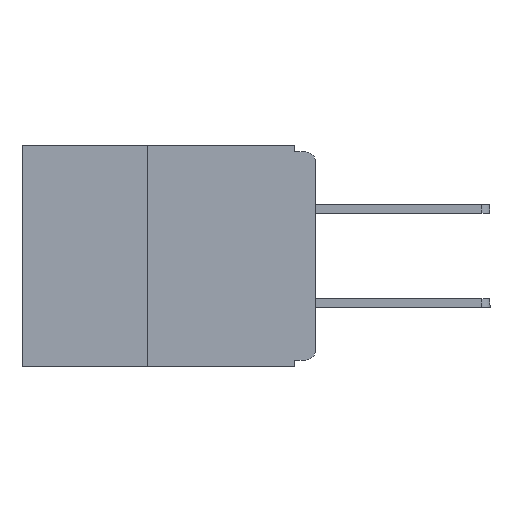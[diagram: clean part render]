
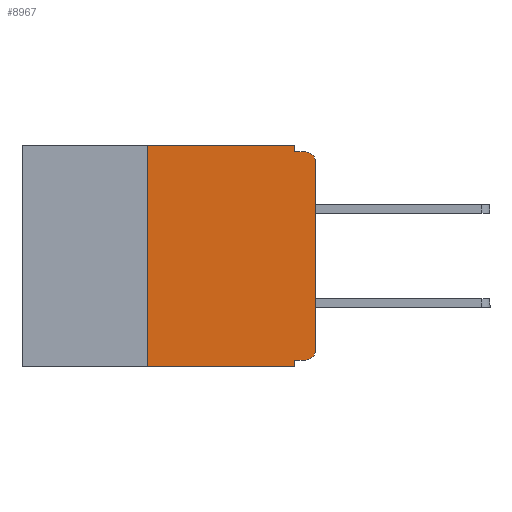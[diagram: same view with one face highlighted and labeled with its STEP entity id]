
A CAD part, left-side view. The second image highlights one B-rep face of the part: STEP entity #8967.
In plain terms, the highlighted planar face has unit normal (-1, 0, 0).
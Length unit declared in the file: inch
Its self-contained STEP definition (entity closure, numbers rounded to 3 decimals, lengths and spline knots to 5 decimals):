
#3 = VERTEX_POINT ( 'NONE', #2808 ) ;
#94 = DIRECTION ( 'NONE',  ( 0., -1., 0. ) ) ;
#122 = CARTESIAN_POINT ( 'NONE',  ( 0., 0.015, -0.01 ) ) ;
#172 = ORIENTED_EDGE ( 'NONE', *, *, #10908, .F. ) ;
#770 = EDGE_CURVE ( 'NONE', #8113, #10541, #4836, .T. ) ;
#774 = EDGE_CURVE ( 'NONE', #13539, #8169, #15194, .T. ) ;
#824 = CIRCLE ( 'NONE', #11983, 0.015 ) ;
#1179 = VECTOR ( 'NONE', #11630, 39.37008 ) ;
#1197 = EDGE_CURVE ( 'NONE', #11318, #4646, #5446, .T. ) ;
#1811 = VECTOR ( 'NONE', #4163, 39.37008 ) ;
#1827 = CARTESIAN_POINT ( 'NONE',  ( 0., 0.015, -0.32 ) ) ;
#2055 = EDGE_LOOP ( 'NONE', ( #10317, #3755, #13589, #3401, #172, #10776, #5014, #6079, #3906, #14213 ) ) ;
#2727 = CARTESIAN_POINT ( 'NONE',  ( 0., 0.015, -0.305 ) ) ;
#2808 = CARTESIAN_POINT ( 'NONE',  ( 0., 0.031, 0. ) ) ;
#3328 = CARTESIAN_POINT ( 'NONE',  ( 0., 0.031, -0.32 ) ) ;
#3401 = ORIENTED_EDGE ( 'NONE', *, *, #4735, .F. ) ;
#3531 = CARTESIAN_POINT ( 'NONE',  ( 0., 0.25, -0.33 ) ) ;
#3652 = EDGE_CURVE ( 'NONE', #11318, #11875, #12510, .T. ) ;
#3719 = EDGE_CURVE ( 'NONE', #10541, #15832, #824, .T. ) ;
#3755 = ORIENTED_EDGE ( 'NONE', *, *, #3719, .T. ) ;
#3906 = ORIENTED_EDGE ( 'NONE', *, *, #774, .F. ) ;
#4073 = DIRECTION ( 'NONE',  ( 0., 0., -1. ) ) ;
#4163 = DIRECTION ( 'NONE',  ( 0., 0., 1. ) ) ;
#4646 = VERTEX_POINT ( 'NONE', #12710 ) ;
#4735 = EDGE_CURVE ( 'NONE', #3, #14463, #13981, .T. ) ;
#4836 = LINE ( 'NONE', #10159, #1179 ) ;
#5014 = ORIENTED_EDGE ( 'NONE', *, *, #3652, .T. ) ;
#5231 = LINE ( 'NONE', #16571, #11992 ) ;
#5446 = LINE ( 'NONE', #3531, #1811 ) ;
#5982 = EDGE_CURVE ( 'NONE', #8169, #11875, #5231, .T. ) ;
#6079 = ORIENTED_EDGE ( 'NONE', *, *, #5982, .F. ) ;
#6675 = DIRECTION ( 'NONE',  ( 0., 0., -1. ) ) ;
#7108 = CARTESIAN_POINT ( 'NONE',  ( 0., 0., -0.025 ) ) ;
#7160 = CARTESIAN_POINT ( 'NONE',  ( 0., 0.031, 0. ) ) ;
#7494 = CARTESIAN_POINT ( 'NONE',  ( 0., 0., -0.305 ) ) ;
#7818 = CARTESIAN_POINT ( 'NONE',  ( 0., 0.031, -0.01 ) ) ;
#8113 = VERTEX_POINT ( 'NONE', #7494 ) ;
#8169 = VERTEX_POINT ( 'NONE', #3328 ) ;
#8844 = VECTOR ( 'NONE', #9784, 39.37008 ) ;
#8901 = VECTOR ( 'NONE', #9251, 39.37008 ) ;
#8906 = LINE ( 'NONE', #16285, #15675 ) ;
#8967 = ADVANCED_FACE ( 'NONE', ( #17340 ), #14447, .F. ) ;
#9251 = DIRECTION ( 'NONE',  ( 0., -1., 0. ) ) ;
#9534 = CIRCLE ( 'NONE', #13207, 0.015 ) ;
#9784 = DIRECTION ( 'NONE',  ( 0., 1., 0. ) ) ;
#9944 = VECTOR ( 'NONE', #6675, 39.37008 ) ;
#10095 = DIRECTION ( 'NONE',  ( 0., -1., 0. ) ) ;
#10159 = CARTESIAN_POINT ( 'NONE',  ( 0., 0., 0. ) ) ;
#10317 = ORIENTED_EDGE ( 'NONE', *, *, #770, .T. ) ;
#10467 = AXIS2_PLACEMENT_3D ( 'NONE', #14852, #14054, #14014 ) ;
#10541 = VERTEX_POINT ( 'NONE', #7108 ) ;
#10776 = ORIENTED_EDGE ( 'NONE', *, *, #1197, .F. ) ;
#10908 = EDGE_CURVE ( 'NONE', #4646, #3, #8906, .T. ) ;
#11052 = CARTESIAN_POINT ( 'NONE',  ( 0., 0.015, -0.025 ) ) ;
#11318 = VERTEX_POINT ( 'NONE', #13174 ) ;
#11333 = VECTOR ( 'NONE', #10095, 39.37008 ) ;
#11450 = DIRECTION ( 'NONE',  ( -1., 0., 0. ) ) ;
#11522 = CARTESIAN_POINT ( 'NONE',  ( 0., 0.031, -0.33 ) ) ;
#11573 = EDGE_CURVE ( 'NONE', #13539, #8113, #9534, .T. ) ;
#11630 = DIRECTION ( 'NONE',  ( 0., 0., 1. ) ) ;
#11661 = DIRECTION ( 'NONE',  ( 0., 0., -1. ) ) ;
#11745 = LINE ( 'NONE', #12823, #11333 ) ;
#11770 = CARTESIAN_POINT ( 'NONE',  ( 0., 0., -0.32 ) ) ;
#11875 = VERTEX_POINT ( 'NONE', #11522 ) ;
#11983 = AXIS2_PLACEMENT_3D ( 'NONE', #11052, #11450, #11661 ) ;
#11992 = VECTOR ( 'NONE', #16632, 39.37008 ) ;
#12200 = DIRECTION ( 'NONE',  ( -1., 0., 0. ) ) ;
#12364 = CARTESIAN_POINT ( 'NONE',  ( 0., 0.437, -0.33 ) ) ;
#12510 = LINE ( 'NONE', #12364, #8901 ) ;
#12710 = CARTESIAN_POINT ( 'NONE',  ( 0., 0.25, 0. ) ) ;
#12823 = CARTESIAN_POINT ( 'NONE',  ( 0., 0., -0.01 ) ) ;
#13174 = CARTESIAN_POINT ( 'NONE',  ( 0., 0.25, -0.33 ) ) ;
#13207 = AXIS2_PLACEMENT_3D ( 'NONE', #2727, #12200, #4073 ) ;
#13539 = VERTEX_POINT ( 'NONE', #1827 ) ;
#13589 = ORIENTED_EDGE ( 'NONE', *, *, #15389, .F. ) ;
#13981 = LINE ( 'NONE', #7160, #9944 ) ;
#14014 = DIRECTION ( 'NONE',  ( 0., 0., -1. ) ) ;
#14054 = DIRECTION ( 'NONE',  ( 1., 0., 0. ) ) ;
#14213 = ORIENTED_EDGE ( 'NONE', *, *, #11573, .T. ) ;
#14447 = PLANE ( 'NONE',  #10467 ) ;
#14463 = VERTEX_POINT ( 'NONE', #7818 ) ;
#14852 = CARTESIAN_POINT ( 'NONE',  ( 0., 0.437, 0. ) ) ;
#15194 = LINE ( 'NONE', #11770, #8844 ) ;
#15389 = EDGE_CURVE ( 'NONE', #14463, #15832, #11745, .T. ) ;
#15675 = VECTOR ( 'NONE', #94, 39.37008 ) ;
#15832 = VERTEX_POINT ( 'NONE', #122 ) ;
#16285 = CARTESIAN_POINT ( 'NONE',  ( 0., 0.437, 0. ) ) ;
#16571 = CARTESIAN_POINT ( 'NONE',  ( 0., 0.031, -0.33 ) ) ;
#16632 = DIRECTION ( 'NONE',  ( 0., 0., -1. ) ) ;
#17340 = FACE_OUTER_BOUND ( 'NONE', #2055, .T. ) ;
